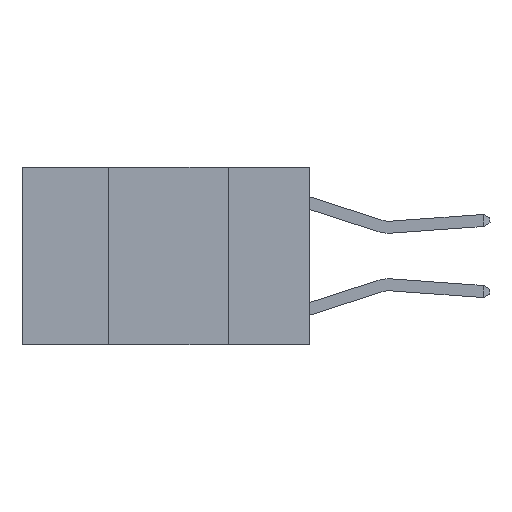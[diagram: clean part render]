
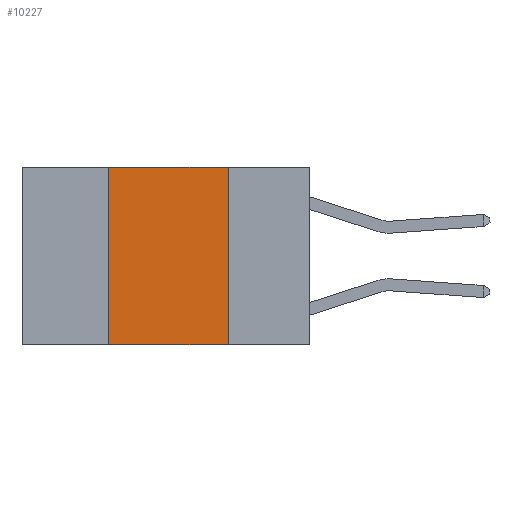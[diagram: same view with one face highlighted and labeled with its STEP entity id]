
A CAD part, left-side view. The second image highlights one B-rep face of the part: STEP entity #10227.
In plain terms, the highlighted planar face has unit normal (-1, 0, 0).
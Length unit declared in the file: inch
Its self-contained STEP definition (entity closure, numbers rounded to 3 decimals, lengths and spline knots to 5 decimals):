
#913 = CARTESIAN_POINT ( 'NONE',  ( 0., 0.6, 0. ) ) ;
#1658 = VERTEX_POINT ( 'NONE', #21630 ) ;
#2973 = LINE ( 'NONE', #913, #7587 ) ;
#3003 = VERTEX_POINT ( 'NONE', #9681 ) ;
#3218 = AXIS2_PLACEMENT_3D ( 'NONE', #12067, #8732, #20490 ) ;
#3680 = FACE_OUTER_BOUND ( 'NONE', #5214, .T. ) ;
#3952 = LINE ( 'NONE', #7581, #7999 ) ;
#5214 = EDGE_LOOP ( 'NONE', ( #11601, #8908, #15435, #18763 ) ) ;
#5613 = DIRECTION ( 'NONE',  ( 0., -1., 0. ) ) ;
#6811 = LINE ( 'NONE', #8281, #19204 ) ;
#7581 = CARTESIAN_POINT ( 'NONE',  ( 0., 0.17, 0. ) ) ;
#7587 = VECTOR ( 'NONE', #14623, 39.37008 ) ;
#7999 = VECTOR ( 'NONE', #9249, 39.37008 ) ;
#8281 = CARTESIAN_POINT ( 'NONE',  ( 0., 0.42, 0. ) ) ;
#8732 = DIRECTION ( 'NONE',  ( 1., 0., 0. ) ) ;
#8908 = ORIENTED_EDGE ( 'NONE', *, *, #9848, .F. ) ;
#9249 = DIRECTION ( 'NONE',  ( 0., 0., -1. ) ) ;
#9681 = CARTESIAN_POINT ( 'NONE',  ( 0., 0.17, -0.37 ) ) ;
#9848 = EDGE_CURVE ( 'NONE', #1658, #18502, #2973, .T. ) ;
#9959 = DIRECTION ( 'NONE',  ( 0., 0., 1. ) ) ;
#10227 = ADVANCED_FACE ( 'NONE', ( #3680 ), #18833, .F. ) ;
#10372 = CARTESIAN_POINT ( 'NONE',  ( 0., 0.42, -0.37 ) ) ;
#11601 = ORIENTED_EDGE ( 'NONE', *, *, #20542, .F. ) ;
#12047 = CARTESIAN_POINT ( 'NONE',  ( 0., 0.17, 0. ) ) ;
#12067 = CARTESIAN_POINT ( 'NONE',  ( 0., 0.6, 0. ) ) ;
#13880 = VECTOR ( 'NONE', #5613, 39.37008 ) ;
#14085 = CARTESIAN_POINT ( 'NONE',  ( 0., 0.6, -0.37 ) ) ;
#14623 = DIRECTION ( 'NONE',  ( 0., -1., 0. ) ) ;
#15435 = ORIENTED_EDGE ( 'NONE', *, *, #18334, .F. ) ;
#15981 = VERTEX_POINT ( 'NONE', #10372 ) ;
#16089 = EDGE_CURVE ( 'NONE', #15981, #3003, #18346, .T. ) ;
#18334 = EDGE_CURVE ( 'NONE', #15981, #1658, #6811, .T. ) ;
#18346 = LINE ( 'NONE', #14085, #13880 ) ;
#18502 = VERTEX_POINT ( 'NONE', #12047 ) ;
#18763 = ORIENTED_EDGE ( 'NONE', *, *, #16089, .T. ) ;
#18833 = PLANE ( 'NONE',  #3218 ) ;
#19204 = VECTOR ( 'NONE', #9959, 39.37008 ) ;
#20490 = DIRECTION ( 'NONE',  ( 0., 0., -1. ) ) ;
#20542 = EDGE_CURVE ( 'NONE', #18502, #3003, #3952, .T. ) ;
#21630 = CARTESIAN_POINT ( 'NONE',  ( 0., 0.42, 0. ) ) ;
